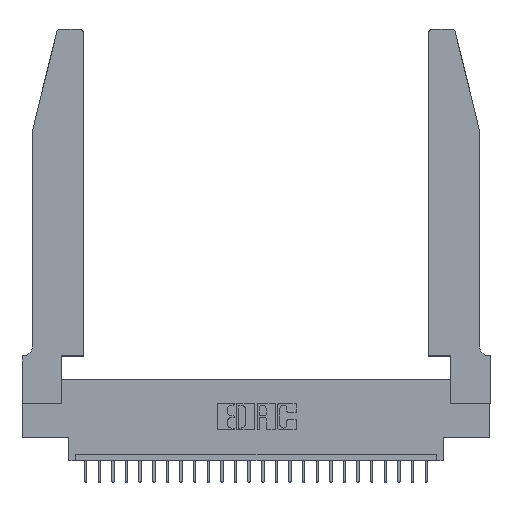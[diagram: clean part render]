
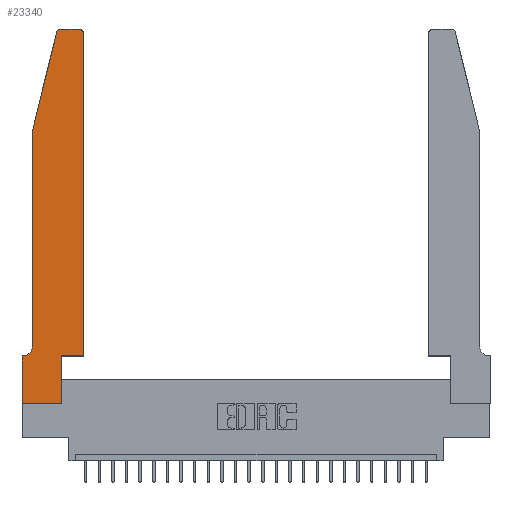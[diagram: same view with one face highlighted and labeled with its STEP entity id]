
A CAD part, top view. The second image highlights one B-rep face of the part: STEP entity #23340.
In plain terms, the highlighted planar face has unit normal (0, 0, 1).
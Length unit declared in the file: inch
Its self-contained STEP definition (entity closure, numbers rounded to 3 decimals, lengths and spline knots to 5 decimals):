
#385 = CARTESIAN_POINT ( 'NONE',  ( 0.4205, 2.75, 0.37 ) ) ;
#613 = ORIENTED_EDGE ( 'NONE', *, *, #19203, .T. ) ;
#874 = ORIENTED_EDGE ( 'NONE', *, *, #12684, .T. ) ;
#1135 = ORIENTED_EDGE ( 'NONE', *, *, #5788, .T. ) ;
#1147 = VECTOR ( 'NONE', #14818, 39.37008 ) ;
#1179 = CARTESIAN_POINT ( 'NONE',  ( 0.4505, 0.35, 0.37 ) ) ;
#1285 = DIRECTION ( 'NONE',  ( 0., -1., 0. ) ) ;
#1286 = CARTESIAN_POINT ( 'NONE',  ( 0.4505, 0.35, 0.37 ) ) ;
#1963 = LINE ( 'NONE', #13085, #8761 ) ;
#2060 = LINE ( 'NONE', #22418, #24881 ) ;
#2116 = EDGE_CURVE ( 'NONE', #17060, #5207, #17585, .T. ) ;
#2273 = ORIENTED_EDGE ( 'NONE', *, *, #4131, .T. ) ;
#2346 = CARTESIAN_POINT ( 'NONE',  ( 0.2865, 0.35, 0.37 ) ) ;
#2513 = PLANE ( 'NONE',  #17745 ) ;
#3609 = LINE ( 'NONE', #11458, #11040 ) ;
#3945 = AXIS2_PLACEMENT_3D ( 'NONE', #20789, #26710, #20887 ) ;
#4131 = EDGE_CURVE ( 'NONE', #20900, #9001, #2060, .T. ) ;
#4341 = CARTESIAN_POINT ( 'NONE',  ( 0.4505, 2.72, 0.37 ) ) ;
#4538 = AXIS2_PLACEMENT_3D ( 'NONE', #21343, #25451, #25726 ) ;
#4711 = DIRECTION ( 'NONE',  ( 1., 0., 0. ) ) ;
#5103 = DIRECTION ( 'NONE',  ( 1., 0., 0. ) ) ;
#5207 = VERTEX_POINT ( 'NONE', #19277 ) ;
#5318 = DIRECTION ( 'NONE',  ( 1., 0., 0. ) ) ;
#5788 = EDGE_CURVE ( 'NONE', #16199, #23217, #14229, .T. ) ;
#6175 = EDGE_CURVE ( 'NONE', #5207, #11491, #22581, .T. ) ;
#6372 = EDGE_CURVE ( 'NONE', #14987, #20638, #3609, .T. ) ;
#6438 = EDGE_CURVE ( 'NONE', #9001, #16199, #1963, .T. ) ;
#7610 = VERTEX_POINT ( 'NONE', #21034 ) ;
#7881 = ORIENTED_EDGE ( 'NONE', *, *, #2116, .T. ) ;
#8185 = EDGE_CURVE ( 'NONE', #7610, #11982, #20251, .T. ) ;
#8728 = ORIENTED_EDGE ( 'NONE', *, *, #6438, .T. ) ;
#8746 = ORIENTED_EDGE ( 'NONE', *, *, #6175, .T. ) ;
#8761 = VECTOR ( 'NONE', #5103, 39.37008 ) ;
#8778 = CARTESIAN_POINT ( 'NONE',  ( 0.284, 2.72, 0.37 ) ) ;
#9001 = VERTEX_POINT ( 'NONE', #2346 ) ;
#9078 = CARTESIAN_POINT ( 'NONE',  ( 0.25487, 2.72718, 0.37 ) ) ;
#9618 = FACE_OUTER_BOUND ( 'NONE', #17719, .T. ) ;
#10258 = CIRCLE ( 'NONE', #3945, 0.03 ) ;
#10711 = VECTOR ( 'NONE', #1285, 39.37008 ) ;
#11015 = DIRECTION ( 'NONE',  ( 0., 0., 1. ) ) ;
#11040 = VECTOR ( 'NONE', #26361, 39.37008 ) ;
#11458 = CARTESIAN_POINT ( 'NONE',  ( 0.2605, 2.75, 0.37 ) ) ;
#11491 = VERTEX_POINT ( 'NONE', #25742 ) ;
#11577 = DIRECTION ( 'NONE',  ( 0., 1., 0. ) ) ;
#11742 = CARTESIAN_POINT ( 'NONE',  ( 0.0755, 0.42, 0.37 ) ) ;
#11982 = VERTEX_POINT ( 'NONE', #11742 ) ;
#12272 = ORIENTED_EDGE ( 'NONE', *, *, #8185, .T. ) ;
#12389 = CARTESIAN_POINT ( 'NONE',  ( 0.0755, 0.35, 0.37 ) ) ;
#12632 = CARTESIAN_POINT ( 'NONE',  ( 0.0755, 2., 0.37 ) ) ;
#12684 = EDGE_CURVE ( 'NONE', #11982, #17060, #17309, .T. ) ;
#12885 = CARTESIAN_POINT ( 'NONE',  ( 0., 0., 0.37 ) ) ;
#13013 = ORIENTED_EDGE ( 'NONE', *, *, #23212, .T. ) ;
#13085 = CARTESIAN_POINT ( 'NONE',  ( 0.4505, 0.35, 0.37 ) ) ;
#13726 = CARTESIAN_POINT ( 'NONE',  ( 0.0055, 0.35, 0.37 ) ) ;
#14229 = LINE ( 'NONE', #1286, #22916 ) ;
#14612 = ORIENTED_EDGE ( 'NONE', *, *, #6372, .T. ) ;
#14736 = VECTOR ( 'NONE', #16298, 39.37008 ) ;
#14818 = DIRECTION ( 'NONE',  ( 1., 0., 0. ) ) ;
#14987 = VERTEX_POINT ( 'NONE', #385 ) ;
#15510 = CARTESIAN_POINT ( 'NONE',  ( 0.284, 2.75, 0.37 ) ) ;
#16199 = VERTEX_POINT ( 'NONE', #1179 ) ;
#16298 = DIRECTION ( 'NONE',  ( 0., -1., 0. ) ) ;
#16397 = EDGE_CURVE ( 'NONE', #20127, #7610, #19934, .T. ) ;
#16847 = DIRECTION ( 'NONE',  ( 0., 1., 0. ) ) ;
#16934 = DIRECTION ( 'NONE',  ( -0.239, -0.971, 0. ) ) ;
#17004 = ORIENTED_EDGE ( 'NONE', *, *, #16397, .T. ) ;
#17037 = VECTOR ( 'NONE', #16934, 39.37008 ) ;
#17060 = VERTEX_POINT ( 'NONE', #13726 ) ;
#17309 = CIRCLE ( 'NONE', #4538, 0.07 ) ;
#17585 = LINE ( 'NONE', #12389, #18222 ) ;
#17586 = LINE ( 'NONE', #12885, #1147 ) ;
#17719 = EDGE_LOOP ( 'NONE', ( #14612, #613, #17004, #12272, #874, #7881, #8746, #20720, #2273, #8728, #1135, #13013 ) ) ;
#17745 = AXIS2_PLACEMENT_3D ( 'NONE', #23001, #11015, #4711 ) ;
#18222 = VECTOR ( 'NONE', #18686, 39.37008 ) ;
#18298 = CARTESIAN_POINT ( 'NONE',  ( 0.0755, 2., 0.37 ) ) ;
#18686 = DIRECTION ( 'NONE',  ( -1., 0., 0. ) ) ;
#19203 = EDGE_CURVE ( 'NONE', #20638, #20127, #23965, .T. ) ;
#19277 = CARTESIAN_POINT ( 'NONE',  ( 0., 0.35, 0.37 ) ) ;
#19934 = LINE ( 'NONE', #12632, #17037 ) ;
#20127 = VERTEX_POINT ( 'NONE', #9078 ) ;
#20251 = LINE ( 'NONE', #18298, #14736 ) ;
#20638 = VERTEX_POINT ( 'NONE', #15510 ) ;
#20720 = ORIENTED_EDGE ( 'NONE', *, *, #25719, .T. ) ;
#20728 = CARTESIAN_POINT ( 'NONE',  ( 0., 0., 0.37 ) ) ;
#20789 = CARTESIAN_POINT ( 'NONE',  ( 0.4205, 2.72, 0.37 ) ) ;
#20887 = DIRECTION ( 'NONE',  ( 1., 0., 0. ) ) ;
#20900 = VERTEX_POINT ( 'NONE', #26242 ) ;
#21034 = CARTESIAN_POINT ( 'NONE',  ( 0.0755, 2., 0.37 ) ) ;
#21343 = CARTESIAN_POINT ( 'NONE',  ( 0.0055, 0.42, 0.37 ) ) ;
#22418 = CARTESIAN_POINT ( 'NONE',  ( 0.2865, 0.35, 0.37 ) ) ;
#22581 = LINE ( 'NONE', #20728, #10711 ) ;
#22916 = VECTOR ( 'NONE', #11577, 39.37008 ) ;
#23001 = CARTESIAN_POINT ( 'NONE',  ( 0., 0.35, 0.37 ) ) ;
#23212 = EDGE_CURVE ( 'NONE', #23217, #14987, #10258, .T. ) ;
#23217 = VERTEX_POINT ( 'NONE', #4341 ) ;
#23340 = ADVANCED_FACE ( 'NONE', ( #9618 ), #2513, .T. ) ;
#23965 = CIRCLE ( 'NONE', #25768, 0.03 ) ;
#24881 = VECTOR ( 'NONE', #16847, 39.37008 ) ;
#25197 = DIRECTION ( 'NONE',  ( 0., 0., 1. ) ) ;
#25451 = DIRECTION ( 'NONE',  ( 0., 0., -1. ) ) ;
#25719 = EDGE_CURVE ( 'NONE', #11491, #20900, #17586, .T. ) ;
#25726 = DIRECTION ( 'NONE',  ( -1., 0., 0. ) ) ;
#25742 = CARTESIAN_POINT ( 'NONE',  ( 0., 0., 0.37 ) ) ;
#25768 = AXIS2_PLACEMENT_3D ( 'NONE', #8778, #25197, #5318 ) ;
#26242 = CARTESIAN_POINT ( 'NONE',  ( 0.2865, 0., 0.37 ) ) ;
#26361 = DIRECTION ( 'NONE',  ( -1., 0., 0. ) ) ;
#26710 = DIRECTION ( 'NONE',  ( 0., 0., 1. ) ) ;
